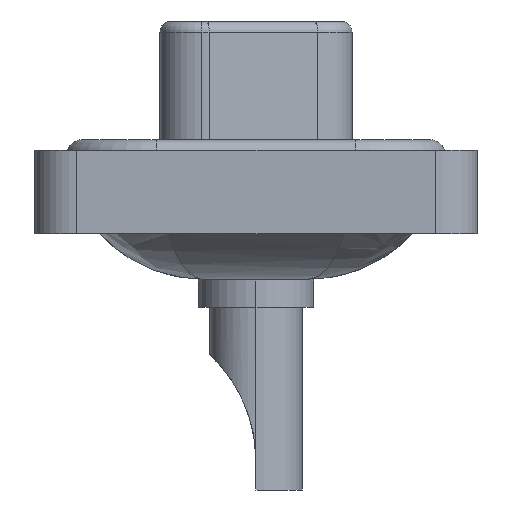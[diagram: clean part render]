
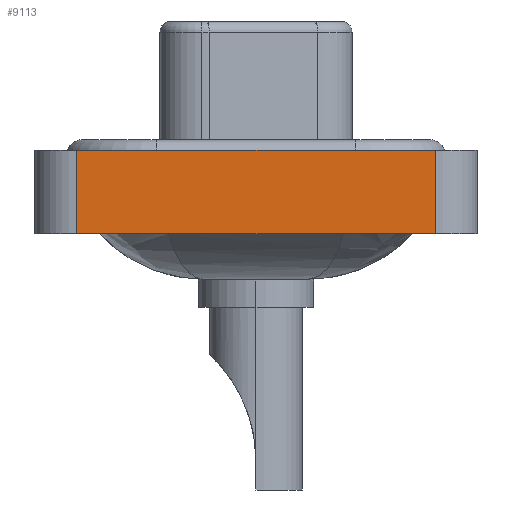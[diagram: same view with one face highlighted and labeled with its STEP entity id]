
A CAD part, left-side view. The second image highlights one B-rep face of the part: STEP entity #9113.
In plain terms, the highlighted planar face has unit normal (-1, 0, 0).
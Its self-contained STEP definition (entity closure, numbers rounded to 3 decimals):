
#488 = ORIENTED_EDGE ( 'NONE', *, *, #12351, .F. ) ;
#1533 = ORIENTED_EDGE ( 'NONE', *, *, #13843, .T. ) ;
#1730 = FACE_OUTER_BOUND ( 'NONE', #15518, .T. ) ;
#2192 = VECTOR ( 'NONE', #5020, 1000. ) ;
#3334 = VERTEX_POINT ( 'NONE', #12954 ) ;
#4788 = ORIENTED_EDGE ( 'NONE', *, *, #10996, .T. ) ;
#5020 = DIRECTION ( 'NONE',  ( 0., -1., 0. ) ) ;
#5069 = CARTESIAN_POINT ( 'NONE',  ( -7.35, -8.55, -3.6 ) ) ;
#5817 = DIRECTION ( 'NONE',  ( 0., -1., 0. ) ) ;
#7495 = AXIS2_PLACEMENT_3D ( 'NONE', #5069, #13481, #14886 ) ;
#7827 = CARTESIAN_POINT ( 'NONE',  ( -7.35, -8.55, -3.6 ) ) ;
#7904 = LINE ( 'NONE', #11652, #10683 ) ;
#9113 = ADVANCED_FACE ( 'NONE', ( #1730 ), #19840, .T. ) ;
#9595 = CARTESIAN_POINT ( 'NONE',  ( -7.35, 8.55, -3.6 ) ) ;
#9651 = VECTOR ( 'NONE', #16199, 1000. ) ;
#10683 = VECTOR ( 'NONE', #17937, 1000. ) ;
#10996 = EDGE_CURVE ( 'NONE', #3334, #14730, #19789, .T. ) ;
#11461 = CARTESIAN_POINT ( 'NONE',  ( -7.35, -8.55, 0.4 ) ) ;
#11588 = ORIENTED_EDGE ( 'NONE', *, *, #19417, .F. ) ;
#11652 = CARTESIAN_POINT ( 'NONE',  ( -7.35, -8.55, -3.6 ) ) ;
#12351 = EDGE_CURVE ( 'NONE', #21142, #12839, #14007, .T. ) ;
#12839 = VERTEX_POINT ( 'NONE', #11461 ) ;
#12916 = VECTOR ( 'NONE', #5817, 1000. ) ;
#12954 = CARTESIAN_POINT ( 'NONE',  ( -7.35, 8.55, -3.6 ) ) ;
#13481 = DIRECTION ( 'NONE',  ( -1., 0., 0. ) ) ;
#13843 = EDGE_CURVE ( 'NONE', #14730, #12839, #7904, .T. ) ;
#14007 = LINE ( 'NONE', #20600, #12916 ) ;
#14103 = CARTESIAN_POINT ( 'NONE',  ( -7.35, -8.55, -3.6 ) ) ;
#14730 = VERTEX_POINT ( 'NONE', #14103 ) ;
#14886 = DIRECTION ( 'NONE',  ( 0., 0., 1. ) ) ;
#15518 = EDGE_LOOP ( 'NONE', ( #1533, #488, #11588, #4788 ) ) ;
#16199 = DIRECTION ( 'NONE',  ( 0., 0., 1. ) ) ;
#17817 = LINE ( 'NONE', #9595, #9651 ) ;
#17937 = DIRECTION ( 'NONE',  ( 0., 0., 1. ) ) ;
#18321 = CARTESIAN_POINT ( 'NONE',  ( -7.35, 8.55, 0.4 ) ) ;
#19417 = EDGE_CURVE ( 'NONE', #3334, #21142, #17817, .T. ) ;
#19789 = LINE ( 'NONE', #7827, #2192 ) ;
#19840 = PLANE ( 'NONE',  #7495 ) ;
#20600 = CARTESIAN_POINT ( 'NONE',  ( -7.35, -8.55, 0.4 ) ) ;
#21142 = VERTEX_POINT ( 'NONE', #18321 ) ;
